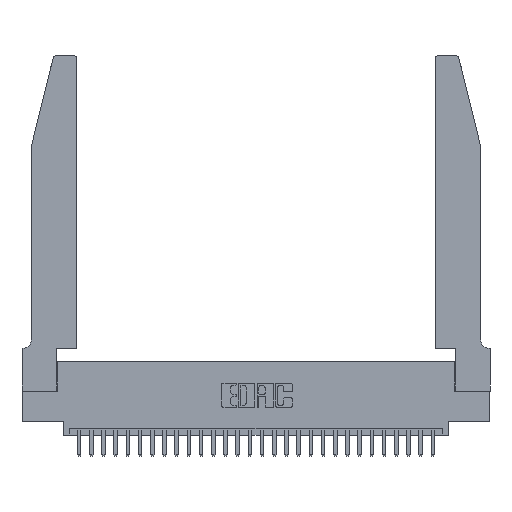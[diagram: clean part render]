
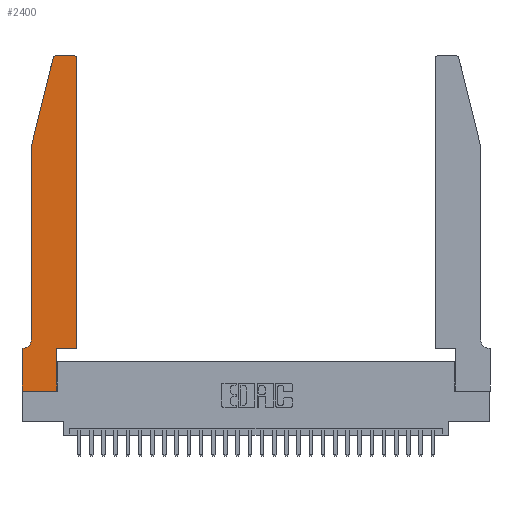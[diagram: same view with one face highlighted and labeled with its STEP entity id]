
A CAD part, top view. The second image highlights one B-rep face of the part: STEP entity #2400.
In plain terms, the highlighted planar face has unit normal (0, 0, 1).
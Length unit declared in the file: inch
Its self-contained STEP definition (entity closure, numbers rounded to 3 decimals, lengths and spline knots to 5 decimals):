
#218 = CARTESIAN_POINT ( 'NONE',  ( 0., 0.35, 0.37 ) ) ;
#294 = VECTOR ( 'NONE', #10912, 39.37008 ) ;
#930 = CARTESIAN_POINT ( 'NONE',  ( 0.284, 2.72, 0.37 ) ) ;
#1020 = DIRECTION ( 'NONE',  ( 0., 0., 1. ) ) ;
#1144 = DIRECTION ( 'NONE',  ( 1., 0., 0. ) ) ;
#1625 = ORIENTED_EDGE ( 'NONE', *, *, #3306, .T. ) ;
#1707 = CARTESIAN_POINT ( 'NONE',  ( 0.284, 2.75, 0.37 ) ) ;
#2160 = CARTESIAN_POINT ( 'NONE',  ( 0.0055, 0.42, 0.37 ) ) ;
#2339 = FACE_OUTER_BOUND ( 'NONE', #17315, .T. ) ;
#2400 = ADVANCED_FACE ( 'NONE', ( #2339 ), #30171, .T. ) ;
#2882 = ORIENTED_EDGE ( 'NONE', *, *, #23671, .T. ) ;
#2938 = VECTOR ( 'NONE', #18649, 39.37008 ) ;
#3280 = CARTESIAN_POINT ( 'NONE',  ( 0.4205, 2.72, 0.37 ) ) ;
#3306 = EDGE_CURVE ( 'NONE', #19755, #28545, #24878, .T. ) ;
#4268 = CARTESIAN_POINT ( 'NONE',  ( 0.4505, 0.35, 0.37 ) ) ;
#4598 = DIRECTION ( 'NONE',  ( 0., 0., 1. ) ) ;
#4928 = EDGE_CURVE ( 'NONE', #8339, #15452, #27312, .T. ) ;
#5008 = LINE ( 'NONE', #10331, #8624 ) ;
#5067 = CARTESIAN_POINT ( 'NONE',  ( 0.0055, 0.35, 0.37 ) ) ;
#6102 = CARTESIAN_POINT ( 'NONE',  ( 0.0755, 2., 0.37 ) ) ;
#7192 = EDGE_CURVE ( 'NONE', #21173, #8339, #25068, .T. ) ;
#7498 = EDGE_CURVE ( 'NONE', #16029, #13589, #5008, .T. ) ;
#7747 = DIRECTION ( 'NONE',  ( 1., 0., 0. ) ) ;
#7967 = LINE ( 'NONE', #14760, #21813 ) ;
#8339 = VERTEX_POINT ( 'NONE', #20347 ) ;
#8354 = VECTOR ( 'NONE', #28727, 39.37008 ) ;
#8576 = CARTESIAN_POINT ( 'NONE',  ( 0.2605, 2.75, 0.37 ) ) ;
#8624 = VECTOR ( 'NONE', #12703, 39.37008 ) ;
#8883 = AXIS2_PLACEMENT_3D ( 'NONE', #3280, #24276, #1144 ) ;
#9365 = CARTESIAN_POINT ( 'NONE',  ( 0.4505, 0.35, 0.37 ) ) ;
#9703 = VECTOR ( 'NONE', #26977, 39.37008 ) ;
#10069 = CARTESIAN_POINT ( 'NONE',  ( 0.25487, 2.72718, 0.37 ) ) ;
#10331 = CARTESIAN_POINT ( 'NONE',  ( 0., 0., 0.37 ) ) ;
#10653 = CARTESIAN_POINT ( 'NONE',  ( 0., 0., 0.37 ) ) ;
#10912 = DIRECTION ( 'NONE',  ( -1., 0., 0. ) ) ;
#11280 = DIRECTION ( 'NONE',  ( 1., 0., 0. ) ) ;
#11406 = DIRECTION ( 'NONE',  ( -1., 0., 0. ) ) ;
#11565 = VECTOR ( 'NONE', #18209, 39.37008 ) ;
#12703 = DIRECTION ( 'NONE',  ( 0., -1., 0. ) ) ;
#13145 = LINE ( 'NONE', #29248, #2938 ) ;
#13309 = CARTESIAN_POINT ( 'NONE',  ( 0.4505, 2.72, 0.37 ) ) ;
#13589 = VERTEX_POINT ( 'NONE', #27792 ) ;
#13605 = EDGE_CURVE ( 'NONE', #28545, #14156, #13145, .T. ) ;
#13820 = EDGE_CURVE ( 'NONE', #27800, #16029, #7967, .T. ) ;
#13862 = EDGE_CURVE ( 'NONE', #14541, #19755, #14894, .T. ) ;
#13961 = AXIS2_PLACEMENT_3D ( 'NONE', #218, #4598, #21159 ) ;
#14156 = VERTEX_POINT ( 'NONE', #21360 ) ;
#14409 = DIRECTION ( 'NONE',  ( -0.239, -0.971, 0. ) ) ;
#14541 = VERTEX_POINT ( 'NONE', #1707 ) ;
#14760 = CARTESIAN_POINT ( 'NONE',  ( 0.0755, 0.35, 0.37 ) ) ;
#14894 = CIRCLE ( 'NONE', #21639, 0.03 ) ;
#15452 = VERTEX_POINT ( 'NONE', #9365 ) ;
#15629 = ORIENTED_EDGE ( 'NONE', *, *, #26850, .T. ) ;
#15660 = CARTESIAN_POINT ( 'NONE',  ( 0.2865, 0.35, 0.37 ) ) ;
#15946 = LINE ( 'NONE', #8576, #294 ) ;
#16029 = VERTEX_POINT ( 'NONE', #24152 ) ;
#16524 = ORIENTED_EDGE ( 'NONE', *, *, #13820, .T. ) ;
#16544 = CIRCLE ( 'NONE', #28637, 0.07 ) ;
#16723 = ORIENTED_EDGE ( 'NONE', *, *, #7498, .T. ) ;
#17315 = EDGE_LOOP ( 'NONE', ( #21953, #17417, #1625, #19612, #15629, #16524, #16723, #22043, #26526, #26083, #2882, #26408 ) ) ;
#17417 = ORIENTED_EDGE ( 'NONE', *, *, #13862, .T. ) ;
#18209 = DIRECTION ( 'NONE',  ( 0., 1., 0. ) ) ;
#18649 = DIRECTION ( 'NONE',  ( 0., -1., 0. ) ) ;
#19341 = CARTESIAN_POINT ( 'NONE',  ( 0.4505, 0.35, 0.37 ) ) ;
#19468 = VERTEX_POINT ( 'NONE', #13309 ) ;
#19612 = ORIENTED_EDGE ( 'NONE', *, *, #13605, .T. ) ;
#19755 = VERTEX_POINT ( 'NONE', #10069 ) ;
#19812 = DIRECTION ( 'NONE',  ( -1., 0., 0. ) ) ;
#20347 = CARTESIAN_POINT ( 'NONE',  ( 0.2865, 0.35, 0.37 ) ) ;
#20636 = LINE ( 'NONE', #10653, #9703 ) ;
#21082 = EDGE_CURVE ( 'NONE', #19468, #21658, #27459, .T. ) ;
#21094 = VECTOR ( 'NONE', #11280, 39.37008 ) ;
#21159 = DIRECTION ( 'NONE',  ( 1., 0., 0. ) ) ;
#21173 = VERTEX_POINT ( 'NONE', #25053 ) ;
#21360 = CARTESIAN_POINT ( 'NONE',  ( 0.0755, 0.42, 0.37 ) ) ;
#21639 = AXIS2_PLACEMENT_3D ( 'NONE', #930, #1020, #7747 ) ;
#21658 = VERTEX_POINT ( 'NONE', #28623 ) ;
#21813 = VECTOR ( 'NONE', #19812, 39.37008 ) ;
#21953 = ORIENTED_EDGE ( 'NONE', *, *, #24628, .T. ) ;
#22043 = ORIENTED_EDGE ( 'NONE', *, *, #28713, .T. ) ;
#23671 = EDGE_CURVE ( 'NONE', #15452, #19468, #24082, .T. ) ;
#24082 = LINE ( 'NONE', #19341, #8354 ) ;
#24152 = CARTESIAN_POINT ( 'NONE',  ( 0., 0.35, 0.37 ) ) ;
#24276 = DIRECTION ( 'NONE',  ( 0., 0., 1. ) ) ;
#24628 = EDGE_CURVE ( 'NONE', #21658, #14541, #15946, .T. ) ;
#24726 = CARTESIAN_POINT ( 'NONE',  ( 0.0755, 2., 0.37 ) ) ;
#24878 = LINE ( 'NONE', #6102, #28875 ) ;
#25053 = CARTESIAN_POINT ( 'NONE',  ( 0.2865, 0., 0.37 ) ) ;
#25068 = LINE ( 'NONE', #15660, #11565 ) ;
#26083 = ORIENTED_EDGE ( 'NONE', *, *, #4928, .T. ) ;
#26408 = ORIENTED_EDGE ( 'NONE', *, *, #21082, .T. ) ;
#26526 = ORIENTED_EDGE ( 'NONE', *, *, #7192, .T. ) ;
#26850 = EDGE_CURVE ( 'NONE', #14156, #27800, #16544, .T. ) ;
#26977 = DIRECTION ( 'NONE',  ( 1., 0., 0. ) ) ;
#27312 = LINE ( 'NONE', #4268, #21094 ) ;
#27459 = CIRCLE ( 'NONE', #8883, 0.03 ) ;
#27792 = CARTESIAN_POINT ( 'NONE',  ( 0., 0., 0.37 ) ) ;
#27800 = VERTEX_POINT ( 'NONE', #5067 ) ;
#28545 = VERTEX_POINT ( 'NONE', #24726 ) ;
#28623 = CARTESIAN_POINT ( 'NONE',  ( 0.4205, 2.75, 0.37 ) ) ;
#28637 = AXIS2_PLACEMENT_3D ( 'NONE', #2160, #29865, #11406 ) ;
#28713 = EDGE_CURVE ( 'NONE', #13589, #21173, #20636, .T. ) ;
#28727 = DIRECTION ( 'NONE',  ( 0., 1., 0. ) ) ;
#28875 = VECTOR ( 'NONE', #14409, 39.37008 ) ;
#29248 = CARTESIAN_POINT ( 'NONE',  ( 0.0755, 2., 0.37 ) ) ;
#29865 = DIRECTION ( 'NONE',  ( 0., 0., -1. ) ) ;
#30171 = PLANE ( 'NONE',  #13961 ) ;
